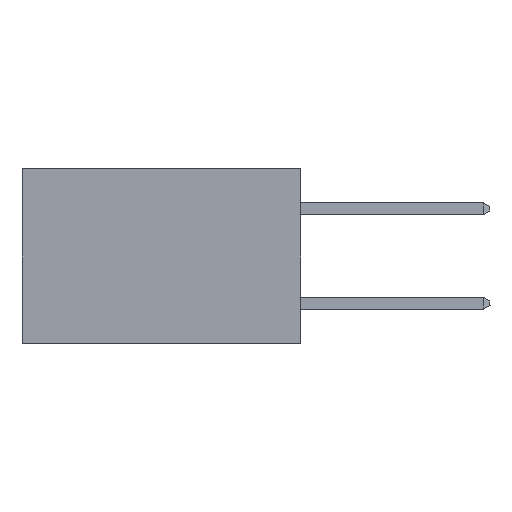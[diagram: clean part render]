
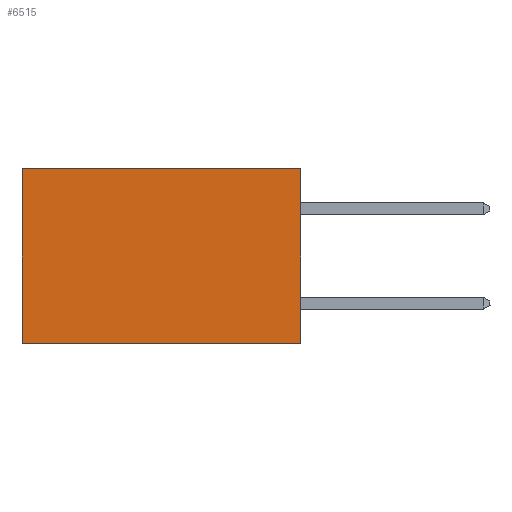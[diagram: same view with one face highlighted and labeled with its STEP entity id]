
A CAD part, left-side view. The second image highlights one B-rep face of the part: STEP entity #6515.
In plain terms, the highlighted planar face has unit normal (-1, 0, 0).
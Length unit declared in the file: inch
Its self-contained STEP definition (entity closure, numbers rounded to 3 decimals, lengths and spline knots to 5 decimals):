
#514 = ORIENTED_EDGE ( 'NONE', *, *, #13585, .F. ) ;
#1224 = VERTEX_POINT ( 'NONE', #4254 ) ;
#1407 = EDGE_LOOP ( 'NONE', ( #21486, #514, #18605, #23002 ) ) ;
#1433 = CARTESIAN_POINT ( 'NONE',  ( 0.277, 0., -0.37 ) ) ;
#1647 = VERTEX_POINT ( 'NONE', #6849 ) ;
#1650 = DIRECTION ( 'NONE',  ( 0., 1., 0. ) ) ;
#2006 = VERTEX_POINT ( 'NONE', #13847 ) ;
#2339 = VECTOR ( 'NONE', #13134, 39.37008 ) ;
#2976 = FACE_OUTER_BOUND ( 'NONE', #1407, .T. ) ;
#4072 = LINE ( 'NONE', #1433, #24060 ) ;
#4254 = CARTESIAN_POINT ( 'NONE',  ( 0.277, 0., 0. ) ) ;
#6187 = VERTEX_POINT ( 'NONE', #15410 ) ;
#6515 = ADVANCED_FACE ( 'NONE', ( #2976 ), #8895, .F. ) ;
#6546 = VECTOR ( 'NONE', #1650, 39.37008 ) ;
#6849 = CARTESIAN_POINT ( 'NONE',  ( 0.277, 0., -0.37 ) ) ;
#8731 = DIRECTION ( 'NONE',  ( 0., 0., -1. ) ) ;
#8781 = DIRECTION ( 'NONE',  ( 1., 0., 0. ) ) ;
#8895 = PLANE ( 'NONE',  #13932 ) ;
#8983 = CARTESIAN_POINT ( 'NONE',  ( 0.277, 0., -0.37 ) ) ;
#10250 = DIRECTION ( 'NONE',  ( 0., 1., 0. ) ) ;
#11103 = LINE ( 'NONE', #13306, #6546 ) ;
#11933 = EDGE_CURVE ( 'NONE', #2006, #6187, #23596, .T. ) ;
#13134 = DIRECTION ( 'NONE',  ( 0., 0., -1. ) ) ;
#13306 = CARTESIAN_POINT ( 'NONE',  ( 0.277, 0., -0.37 ) ) ;
#13585 = EDGE_CURVE ( 'NONE', #1647, #6187, #11103, .T. ) ;
#13847 = CARTESIAN_POINT ( 'NONE',  ( 0.277, 0.59, 0. ) ) ;
#13932 = AXIS2_PLACEMENT_3D ( 'NONE', #8983, #8781, #8731 ) ;
#14815 = EDGE_CURVE ( 'NONE', #1224, #1647, #4072, .T. ) ;
#15410 = CARTESIAN_POINT ( 'NONE',  ( 0.277, 0.59, -0.37 ) ) ;
#17869 = VECTOR ( 'NONE', #10250, 39.37008 ) ;
#18605 = ORIENTED_EDGE ( 'NONE', *, *, #14815, .F. ) ;
#18971 = DIRECTION ( 'NONE',  ( 0., 0., -1. ) ) ;
#19899 = CARTESIAN_POINT ( 'NONE',  ( 0.277, 0., 0. ) ) ;
#19975 = EDGE_CURVE ( 'NONE', #1224, #2006, #22993, .T. ) ;
#21486 = ORIENTED_EDGE ( 'NONE', *, *, #11933, .T. ) ;
#22812 = CARTESIAN_POINT ( 'NONE',  ( 0.277, 0.59, -0.37 ) ) ;
#22993 = LINE ( 'NONE', #19899, #17869 ) ;
#23002 = ORIENTED_EDGE ( 'NONE', *, *, #19975, .T. ) ;
#23596 = LINE ( 'NONE', #22812, #2339 ) ;
#24060 = VECTOR ( 'NONE', #18971, 39.37008 ) ;
